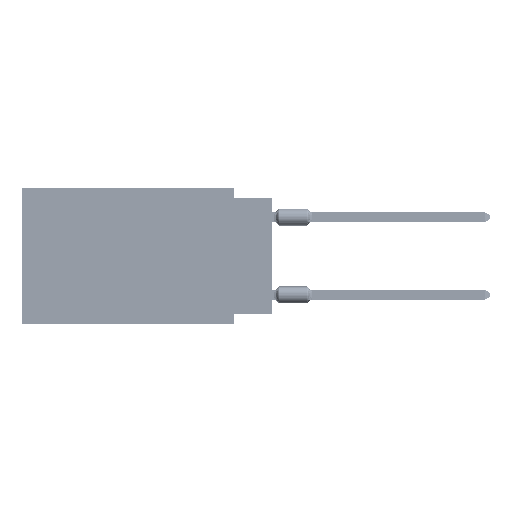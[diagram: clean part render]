
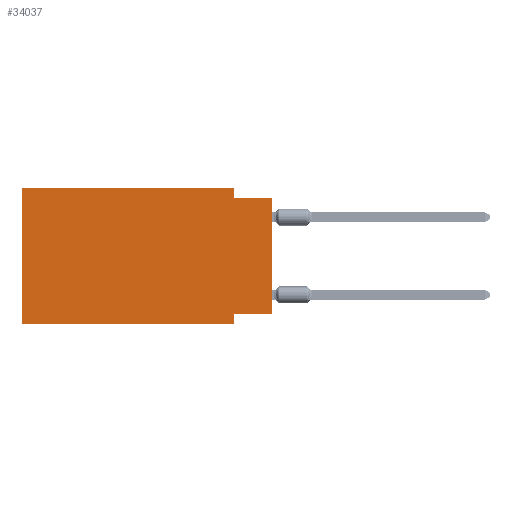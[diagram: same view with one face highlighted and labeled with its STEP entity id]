
A CAD part, left-side view. The second image highlights one B-rep face of the part: STEP entity #34037.
In plain terms, the highlighted planar face has unit normal (-1, 0, 0).
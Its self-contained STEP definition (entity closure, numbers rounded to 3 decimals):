
#638 = LINE ( 'NONE', #34122, #90814 ) ;
#1660 = CARTESIAN_POINT ( 'NONE',  ( 0., 2.54, 0. ) ) ;
#2531 = VECTOR ( 'NONE', #68680, 1000. ) ;
#5297 = LINE ( 'NONE', #101598, #68508 ) ;
#6995 = LINE ( 'NONE', #42181, #2531 ) ;
#9148 = LINE ( 'NONE', #33968, #112810 ) ;
#10357 = CARTESIAN_POINT ( 'NONE',  ( 0., 2.54, -8.255 ) ) ;
#16963 = ORIENTED_EDGE ( 'NONE', *, *, #92097, .F. ) ;
#18828 = CARTESIAN_POINT ( 'NONE',  ( 0., 16.383, -8.89 ) ) ;
#19296 = VERTEX_POINT ( 'NONE', #1660 ) ;
#19728 = AXIS2_PLACEMENT_3D ( 'NONE', #43920, #24926, #51985 ) ;
#24158 = VERTEX_POINT ( 'NONE', #51825 ) ;
#24926 = DIRECTION ( 'NONE',  ( 1., 0., 0. ) ) ;
#26004 = VERTEX_POINT ( 'NONE', #18828 ) ;
#26887 = CARTESIAN_POINT ( 'NONE',  ( 0., 2.54, -8.89 ) ) ;
#27224 = LINE ( 'NONE', #62373, #80294 ) ;
#27836 = ORIENTED_EDGE ( 'NONE', *, *, #92977, .F. ) ;
#28450 = EDGE_CURVE ( 'NONE', #26004, #41627, #6995, .T. ) ;
#31446 = CARTESIAN_POINT ( 'NONE',  ( 0., 0., -0.635 ) ) ;
#33968 = CARTESIAN_POINT ( 'NONE',  ( 0., 0., -8.255 ) ) ;
#34037 = ADVANCED_FACE ( 'NONE', ( #42224 ), #69863, .F. ) ;
#34122 = CARTESIAN_POINT ( 'NONE',  ( 0., 2.54, 0. ) ) ;
#35346 = ORIENTED_EDGE ( 'NONE', *, *, #91504, .F. ) ;
#38380 = LINE ( 'NONE', #31446, #71606 ) ;
#41627 = VERTEX_POINT ( 'NONE', #26887 ) ;
#42181 = CARTESIAN_POINT ( 'NONE',  ( 0., 16.383, -8.89 ) ) ;
#42224 = FACE_OUTER_BOUND ( 'NONE', #86090, .T. ) ;
#42811 = LINE ( 'NONE', #76827, #94982 ) ;
#43920 = CARTESIAN_POINT ( 'NONE',  ( 0., 16.383, 0. ) ) ;
#48737 = DIRECTION ( 'NONE',  ( 0., -1., 0. ) ) ;
#50818 = ORIENTED_EDGE ( 'NONE', *, *, #67500, .F. ) ;
#51825 = CARTESIAN_POINT ( 'NONE',  ( 0., 16.383, 0. ) ) ;
#51985 = DIRECTION ( 'NONE',  ( 0., 0., -1. ) ) ;
#54881 = ORIENTED_EDGE ( 'NONE', *, *, #81844, .F. ) ;
#57836 = CARTESIAN_POINT ( 'NONE',  ( 0., 2.54, -8.89 ) ) ;
#62373 = CARTESIAN_POINT ( 'NONE',  ( 0., 0., 0. ) ) ;
#67481 = CARTESIAN_POINT ( 'NONE',  ( 0., 2.54, -0.635 ) ) ;
#67500 = EDGE_CURVE ( 'NONE', #109386, #96280, #38380, .T. ) ;
#68144 = ORIENTED_EDGE ( 'NONE', *, *, #82175, .T. ) ;
#68508 = VECTOR ( 'NONE', #94655, 1000. ) ;
#68680 = DIRECTION ( 'NONE',  ( 0., -1., 0. ) ) ;
#69843 = DIRECTION ( 'NONE',  ( 0., 0., -1. ) ) ;
#69863 = PLANE ( 'NONE',  #19728 ) ;
#71590 = DIRECTION ( 'NONE',  ( 0., 0., 1. ) ) ;
#71606 = VECTOR ( 'NONE', #48737, 1000. ) ;
#71671 = ORIENTED_EDGE ( 'NONE', *, *, #112275, .F. ) ;
#76827 = CARTESIAN_POINT ( 'NONE',  ( 0., 16.383, 0. ) ) ;
#80294 = VECTOR ( 'NONE', #71590, 1000. ) ;
#81844 = EDGE_CURVE ( 'NONE', #113987, #41627, #93582, .T. ) ;
#82175 = EDGE_CURVE ( 'NONE', #89674, #96280, #27224, .T. ) ;
#86090 = EDGE_LOOP ( 'NONE', ( #68144, #50818, #27836, #35346, #71671, #112509, #54881, #16963 ) ) ;
#89674 = VERTEX_POINT ( 'NONE', #105203 ) ;
#90814 = VECTOR ( 'NONE', #69843, 1000. ) ;
#91504 = EDGE_CURVE ( 'NONE', #24158, #19296, #5297, .T. ) ;
#92097 = EDGE_CURVE ( 'NONE', #89674, #113987, #9148, .T. ) ;
#92977 = EDGE_CURVE ( 'NONE', #19296, #109386, #638, .T. ) ;
#93018 = DIRECTION ( 'NONE',  ( 0., 0., -1. ) ) ;
#93582 = LINE ( 'NONE', #57836, #102280 ) ;
#94655 = DIRECTION ( 'NONE',  ( 0., -1., 0. ) ) ;
#94982 = VECTOR ( 'NONE', #112030, 1000. ) ;
#96280 = VERTEX_POINT ( 'NONE', #105098 ) ;
#101598 = CARTESIAN_POINT ( 'NONE',  ( 0., 16.383, 0. ) ) ;
#102280 = VECTOR ( 'NONE', #93018, 1000. ) ;
#105098 = CARTESIAN_POINT ( 'NONE',  ( 0., 0., -0.635 ) ) ;
#105203 = CARTESIAN_POINT ( 'NONE',  ( 0., 0., -8.255 ) ) ;
#105442 = DIRECTION ( 'NONE',  ( 0., 1., 0. ) ) ;
#109386 = VERTEX_POINT ( 'NONE', #67481 ) ;
#112030 = DIRECTION ( 'NONE',  ( 0., 0., 1. ) ) ;
#112275 = EDGE_CURVE ( 'NONE', #26004, #24158, #42811, .T. ) ;
#112509 = ORIENTED_EDGE ( 'NONE', *, *, #28450, .T. ) ;
#112810 = VECTOR ( 'NONE', #105442, 1000. ) ;
#113987 = VERTEX_POINT ( 'NONE', #10357 ) ;
